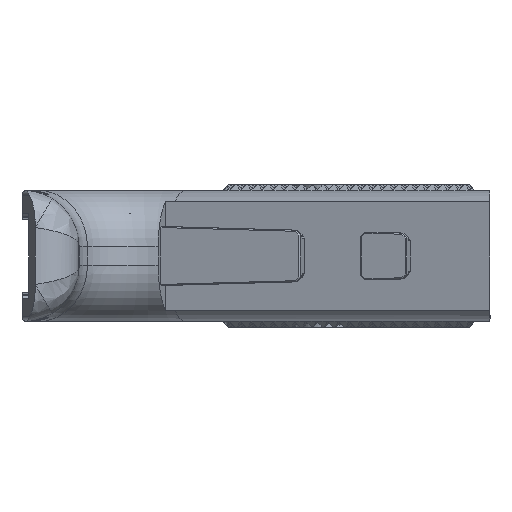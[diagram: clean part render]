
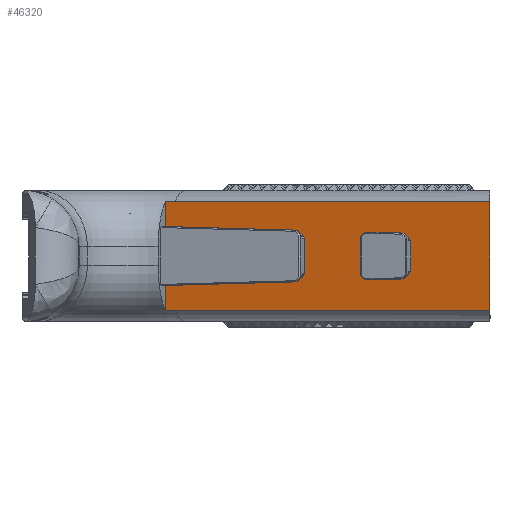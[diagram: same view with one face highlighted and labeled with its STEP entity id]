
A CAD part, left-side view. The second image highlights one B-rep face of the part: STEP entity #46320.
In plain terms, the highlighted planar face has unit normal (-0.951, 0.309, 0).
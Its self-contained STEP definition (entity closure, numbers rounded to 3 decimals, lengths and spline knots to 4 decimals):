
#233=FACE_BOUND('',#6644,.T.);
#597=B_SPLINE_CURVE_WITH_KNOTS('',3,(#88520,#88521,#88522,#88523,#88524,
#88525,#88526),.UNSPECIFIED.,.F.,.F.,(4,3,4),(0.,0.1181,0.2155),
 .UNSPECIFIED.);
#598=B_SPLINE_CURVE_WITH_KNOTS('',3,(#88534,#88535,#88536,#88537,#88538,
#88539,#88540),.UNSPECIFIED.,.F.,.F.,(4,3,4),(-0.2155,-0.1181,
0.),.UNSPECIFIED.);
#3644=FACE_OUTER_BOUND('',#6643,.T.);
#6643=EDGE_LOOP('',(#38767,#38768,#38769,#38770,#38771,#38772,#38773,#38774,
#38775,#38776,#38777,#38778));
#6644=EDGE_LOOP('',(#38779,#38780,#38781,#38782,#38783,#38784,#38785,#38786,
#38787));
#11839=LINE('',#88409,#17378);
#11857=LINE('',#88447,#17396);
#11865=LINE('',#88464,#17404);
#11870=LINE('',#88473,#17409);
#11872=LINE('',#88476,#17411);
#11874=LINE('',#88481,#17413);
#11876=LINE('',#88485,#17415);
#11878=LINE('',#88488,#17417);
#11880=LINE('',#88492,#17419);
#11881=LINE('',#88494,#17420);
#11887=LINE('',#88507,#17426);
#11889=LINE('',#88511,#17428);
#11890=LINE('',#88514,#17429);
#11892=LINE('',#88518,#17431);
#11893=LINE('',#88528,#17432);
#11894=LINE('',#88530,#17433);
#11895=LINE('',#88532,#17434);
#11896=LINE('',#88542,#17435);
#11897=LINE('',#88543,#17436);
#17378=VECTOR('',#60131,0.3937);
#17396=VECTOR('',#60167,0.3937);
#17404=VECTOR('',#60181,0.3937);
#17409=VECTOR('',#60190,0.3937);
#17411=VECTOR('',#60194,0.3937);
#17413=VECTOR('',#60198,0.3937);
#17415=VECTOR('',#60202,0.3937);
#17417=VECTOR('',#60206,0.3937);
#17419=VECTOR('',#60210,0.3937);
#17420=VECTOR('',#60213,0.3937);
#17426=VECTOR('',#60229,0.3937);
#17428=VECTOR('',#60233,0.3937);
#17429=VECTOR('',#60236,0.3937);
#17431=VECTOR('',#60240,0.3937);
#17432=VECTOR('',#60241,0.3937);
#17433=VECTOR('',#60242,0.3937);
#17434=VECTOR('',#60243,0.3937);
#17435=VECTOR('',#60244,0.3937);
#17436=VECTOR('',#60245,0.3937);
#21120=VERTEX_POINT('',#88406);
#21121=VERTEX_POINT('',#88408);
#21131=VERTEX_POINT('',#88444);
#21132=VERTEX_POINT('',#88446);
#21137=VERTEX_POINT('',#88461);
#21138=VERTEX_POINT('',#88463);
#21140=VERTEX_POINT('',#88472);
#21141=VERTEX_POINT('',#88478);
#21142=VERTEX_POINT('',#88480);
#21143=VERTEX_POINT('',#88484);
#21144=VERTEX_POINT('',#88490);
#21146=VERTEX_POINT('',#88505);
#21147=VERTEX_POINT('',#88509);
#21148=VERTEX_POINT('',#88513);
#21149=VERTEX_POINT('',#88517);
#21150=VERTEX_POINT('',#88519);
#21151=VERTEX_POINT('',#88527);
#21152=VERTEX_POINT('',#88529);
#21153=VERTEX_POINT('',#88531);
#21154=VERTEX_POINT('',#88533);
#21155=VERTEX_POINT('',#88541);
#27123=EDGE_CURVE('',#21121,#21120,#11839,.T.);
#27141=EDGE_CURVE('',#21131,#21132,#11857,.T.);
#27149=EDGE_CURVE('',#21137,#21138,#11865,.F.);
#27154=EDGE_CURVE('',#21121,#21140,#11870,.F.);
#27156=EDGE_CURVE('',#21137,#21140,#11872,.T.);
#27158=EDGE_CURVE('',#21141,#21142,#11874,.F.);
#27160=EDGE_CURVE('',#21143,#21142,#11876,.T.);
#27162=EDGE_CURVE('',#21141,#21138,#11878,.T.);
#27164=EDGE_CURVE('',#21144,#21120,#11880,.F.);
#27165=EDGE_CURVE('',#21143,#21144,#11881,.F.);
#27171=EDGE_CURVE('',#21146,#21131,#11887,.F.);
#27173=EDGE_CURVE('',#21146,#21147,#11889,.T.);
#27174=EDGE_CURVE('',#21132,#21148,#11890,.F.);
#27176=EDGE_CURVE('',#21149,#21147,#11892,.T.);
#27177=EDGE_CURVE('',#21150,#21149,#597,.T.);
#27178=EDGE_CURVE('',#21151,#21150,#11893,.T.);
#27179=EDGE_CURVE('',#21152,#21151,#11894,.T.);
#27180=EDGE_CURVE('',#21153,#21152,#11895,.T.);
#27181=EDGE_CURVE('',#21154,#21153,#598,.T.);
#27182=EDGE_CURVE('',#21155,#21154,#11896,.T.);
#27183=EDGE_CURVE('',#21155,#21148,#11897,.T.);
#38767=ORIENTED_EDGE('',*,*,#27173,.T.);
#38768=ORIENTED_EDGE('',*,*,#27176,.F.);
#38769=ORIENTED_EDGE('',*,*,#27177,.F.);
#38770=ORIENTED_EDGE('',*,*,#27178,.F.);
#38771=ORIENTED_EDGE('',*,*,#27179,.F.);
#38772=ORIENTED_EDGE('',*,*,#27180,.F.);
#38773=ORIENTED_EDGE('',*,*,#27181,.F.);
#38774=ORIENTED_EDGE('',*,*,#27182,.F.);
#38775=ORIENTED_EDGE('',*,*,#27183,.T.);
#38776=ORIENTED_EDGE('',*,*,#27174,.F.);
#38777=ORIENTED_EDGE('',*,*,#27141,.F.);
#38778=ORIENTED_EDGE('',*,*,#27171,.F.);
#38779=ORIENTED_EDGE('',*,*,#27123,.T.);
#38780=ORIENTED_EDGE('',*,*,#27164,.F.);
#38781=ORIENTED_EDGE('',*,*,#27165,.F.);
#38782=ORIENTED_EDGE('',*,*,#27160,.T.);
#38783=ORIENTED_EDGE('',*,*,#27158,.F.);
#38784=ORIENTED_EDGE('',*,*,#27162,.T.);
#38785=ORIENTED_EDGE('',*,*,#27149,.F.);
#38786=ORIENTED_EDGE('',*,*,#27156,.T.);
#38787=ORIENTED_EDGE('',*,*,#27154,.F.);
#43503=PLANE('',#49424);
#46320=ADVANCED_FACE('',(#3644,#233),#43503,.T.);
#49424=AXIS2_PLACEMENT_3D('',#88516,#60238,#60239);
#60131=DIRECTION('',(0.,0.,1.));
#60167=DIRECTION('',(0.,0.,1.));
#60181=DIRECTION('',(0.216,0.664,-0.716));
#60190=DIRECTION('',(0.221,0.681,0.698));
#60194=DIRECTION('',(0.309,0.951,-0.026));
#60198=DIRECTION('',(-0.216,-0.664,-0.716));
#60202=DIRECTION('',(-0.309,-0.951,-0.026));
#60206=DIRECTION('',(0.,0.,-1.));
#60210=DIRECTION('',(-0.12,-0.37,0.921));
#60213=DIRECTION('',(-0.221,-0.681,0.698));
#60229=DIRECTION('',(0.216,0.664,-0.716));
#60233=DIRECTION('',(0.309,0.951,-0.026));
#60236=DIRECTION('',(-0.216,-0.664,-0.716));
#60238=DIRECTION('center_axis',(-0.951,0.309,0.));
#60239=DIRECTION('ref_axis',(0.,0.,
1.));
#60240=DIRECTION('',(0.,0.,1.));
#60241=DIRECTION('',(0.309,0.951,0.));
#60242=DIRECTION('',(0.,0.,-1.));
#60243=DIRECTION('',(-0.309,-0.951,0.));
#60244=DIRECTION('',(0.,0.,1.));
#60245=DIRECTION('',(-0.309,-0.951,-0.026));
#88406=CARTESIAN_POINT('',(-2.8962,-0.8838,-0.6352));
#88408=CARTESIAN_POINT('',(-2.8962,-0.8838,-0.9101));
#88409=CARTESIAN_POINT('',(-2.8962,-0.8838,-0.7677));
#88444=CARTESIAN_POINT('',(-2.7262,-0.3607,-0.9245));
#88446=CARTESIAN_POINT('',(-2.7262,-0.3607,-0.6109));
#88447=CARTESIAN_POINT('',(-2.7262,-0.3607,-0.9154));
#88461=CARTESIAN_POINT('',(-3.0247,-1.2792,-0.909));
#88463=CARTESIAN_POINT('',(-3.0277,-1.2886,-0.8989));
#88464=CARTESIAN_POINT('',(-2.9908,-1.1749,-1.0217));
#88472=CARTESIAN_POINT('',(-2.8992,-0.8932,-0.9197));
#88473=CARTESIAN_POINT('',(-2.8709,-0.806,-0.8303));
#88476=CARTESIAN_POINT('',(-3.0469,-1.3476,-0.9072));
#88478=CARTESIAN_POINT('',(-3.0277,-1.2886,-0.6365));
#88480=CARTESIAN_POINT('',(-3.0247,-1.2792,-0.6264));
#88481=CARTESIAN_POINT('',(-2.9908,-1.1749,-0.5138));
#88484=CARTESIAN_POINT('',(-2.8992,-0.8932,-0.6158));
#88485=CARTESIAN_POINT('',(-3.0469,-1.3476,-0.6283));
#88488=CARTESIAN_POINT('',(-3.0277,-1.2886,-0.899));
#88490=CARTESIAN_POINT('',(-2.8984,-0.8905,-0.6185));
#88492=CARTESIAN_POINT('',(-2.885,-0.8493,-0.7213));
#88494=CARTESIAN_POINT('',(-2.8709,-0.806,-0.7051));
#88505=CARTESIAN_POINT('',(-2.7232,-0.3514,-0.9346));
#88507=CARTESIAN_POINT('',(-2.7647,-0.479,-0.7968));
#88509=CARTESIAN_POINT('',(-2.3324,0.8513,-0.9677));
#88511=CARTESIAN_POINT('',(-3.0469,-1.3476,-0.9072));
#88513=CARTESIAN_POINT('',(-2.7232,-0.3514,-0.6008));
#88514=CARTESIAN_POINT('',(-2.7647,-0.479,-0.7386));
#88516=CARTESIAN_POINT('Origin',(-2.8375,-0.7031,-0.7677));
#88517=CARTESIAN_POINT('',(-2.3324,0.8513,-1.2459));
#88518=CARTESIAN_POINT('',(-2.3324,0.8513,-1.0302));
#88519=CARTESIAN_POINT('',(-2.3592,0.7689,-1.2425));
#88520=CARTESIAN_POINT('Ctrl Pts',(-2.3592,0.7689,
-1.2425));
#88521=CARTESIAN_POINT('Ctrl Pts',(-2.3544,0.7836,
-1.2425));
#88522=CARTESIAN_POINT('Ctrl Pts',(-2.3495,0.7986,
-1.2428));
#88523=CARTESIAN_POINT('Ctrl Pts',(-2.3446,0.8138,
-1.2435));
#88524=CARTESIAN_POINT('Ctrl Pts',(-2.3405,0.8264,
-1.2441));
#88525=CARTESIAN_POINT('Ctrl Pts',(-2.3365,0.8388,
-1.2449));
#88526=CARTESIAN_POINT('Ctrl Pts',(-2.3324,0.8513,-1.2459));
#88527=CARTESIAN_POINT('',(-3.2516,-1.9775,-1.2425));
#88528=CARTESIAN_POINT('',(-2.1969,1.2684,-1.2425));
#88529=CARTESIAN_POINT('',(-3.2516,-1.9775,-0.2929));
#88530=CARTESIAN_POINT('',(-3.2516,-1.9775,-0.3839));
#88531=CARTESIAN_POINT('',(-2.3592,0.7689,-0.2929));
#88532=CARTESIAN_POINT('',(-2.6906,-0.2509,-0.2929));
#88533=CARTESIAN_POINT('',(-2.3324,0.8513,-0.2895));
#88534=CARTESIAN_POINT('Ctrl Pts',(-2.3324,0.8513,-0.2895));
#88535=CARTESIAN_POINT('Ctrl Pts',(-2.3365,0.8388,
-0.2905));
#88536=CARTESIAN_POINT('Ctrl Pts',(-2.3405,0.8264,
-0.2913));
#88537=CARTESIAN_POINT('Ctrl Pts',(-2.3446,0.8138,
-0.2919));
#88538=CARTESIAN_POINT('Ctrl Pts',(-2.3495,0.7986,
-0.2926));
#88539=CARTESIAN_POINT('Ctrl Pts',(-2.3544,0.7836,
-0.2929));
#88540=CARTESIAN_POINT('Ctrl Pts',(-2.3592,0.7689,
-0.2929));
#88541=CARTESIAN_POINT('',(-2.3324,0.8513,-0.5677));
#88542=CARTESIAN_POINT('',(-2.3324,0.8513,-0.7677));
#88543=CARTESIAN_POINT('',(-3.0469,-1.3476,-0.6283));
